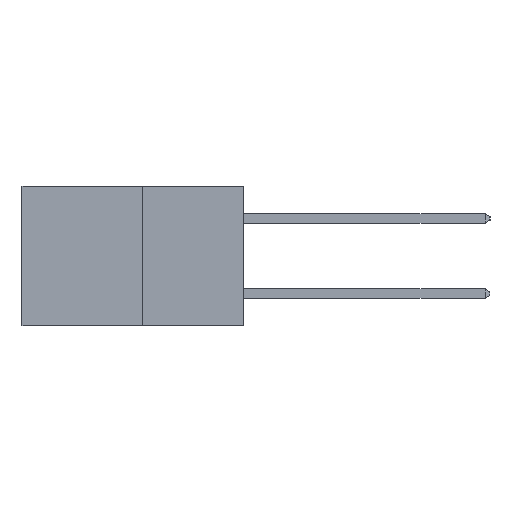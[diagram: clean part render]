
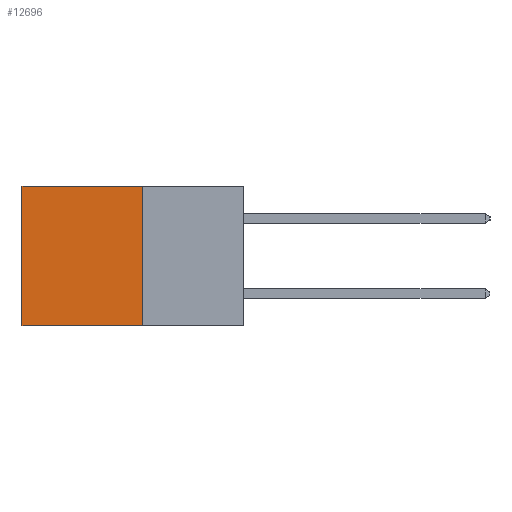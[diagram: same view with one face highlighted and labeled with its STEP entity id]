
A CAD part, left-side view. The second image highlights one B-rep face of the part: STEP entity #12696.
In plain terms, the highlighted planar face has unit normal (-1, 0, 0).
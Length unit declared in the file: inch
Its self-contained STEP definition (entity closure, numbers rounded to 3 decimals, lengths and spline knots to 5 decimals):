
#537 = CARTESIAN_POINT ( 'NONE',  ( 0.277, 0.27, 0. ) ) ;
#1499 = CARTESIAN_POINT ( 'NONE',  ( 0.277, 0.27, -0.37 ) ) ;
#1795 = VERTEX_POINT ( 'NONE', #537 ) ;
#4181 = VECTOR ( 'NONE', #15242, 39.37008 ) ;
#4326 = VECTOR ( 'NONE', #18595, 39.37008 ) ;
#5209 = PLANE ( 'NONE',  #26498 ) ;
#7525 = DIRECTION ( 'NONE',  ( 1., 0., 0. ) ) ;
#9080 = ORIENTED_EDGE ( 'NONE', *, *, #10311, .F. ) ;
#10311 = EDGE_CURVE ( 'NONE', #29391, #19049, #10317, .T. ) ;
#10317 = LINE ( 'NONE', #1499, #4181 ) ;
#11465 = LINE ( 'NONE', #11926, #23617 ) ;
#11926 = CARTESIAN_POINT ( 'NONE',  ( 0.277, 0.59, -0.37 ) ) ;
#12463 = VERTEX_POINT ( 'NONE', #22441 ) ;
#12664 = CARTESIAN_POINT ( 'NONE',  ( 0.277, 0.27, -0.37 ) ) ;
#12682 = CARTESIAN_POINT ( 'NONE',  ( 0.277, 0.59, -0.37 ) ) ;
#12696 = ADVANCED_FACE ( 'NONE', ( #24678 ), #5209, .F. ) ;
#14214 = DIRECTION ( 'NONE',  ( 0., 0., -1. ) ) ;
#14782 = ORIENTED_EDGE ( 'NONE', *, *, #18132, .T. ) ;
#15242 = DIRECTION ( 'NONE',  ( 0., 1., 0. ) ) ;
#16271 = CARTESIAN_POINT ( 'NONE',  ( 0.277, 0.27, 0. ) ) ;
#16441 = EDGE_CURVE ( 'NONE', #1795, #29391, #26967, .T. ) ;
#17982 = LINE ( 'NONE', #16271, #4326 ) ;
#18132 = EDGE_CURVE ( 'NONE', #12463, #19049, #11465, .T. ) ;
#18595 = DIRECTION ( 'NONE',  ( 0., 1., 0. ) ) ;
#19049 = VERTEX_POINT ( 'NONE', #12682 ) ;
#19786 = CARTESIAN_POINT ( 'NONE',  ( 0.277, 0.27, -0.37 ) ) ;
#21252 = CARTESIAN_POINT ( 'NONE',  ( 0.277, 0.27, -0.37 ) ) ;
#22441 = CARTESIAN_POINT ( 'NONE',  ( 0.277, 0.59, 0. ) ) ;
#23516 = DIRECTION ( 'NONE',  ( 0., 0., -1. ) ) ;
#23617 = VECTOR ( 'NONE', #14214, 39.37008 ) ;
#24276 = EDGE_CURVE ( 'NONE', #1795, #12463, #17982, .T. ) ;
#24374 = EDGE_LOOP ( 'NONE', ( #14782, #9080, #24516, #26384 ) ) ;
#24516 = ORIENTED_EDGE ( 'NONE', *, *, #16441, .F. ) ;
#24678 = FACE_OUTER_BOUND ( 'NONE', #24374, .T. ) ;
#25520 = VECTOR ( 'NONE', #26350, 39.37008 ) ;
#26350 = DIRECTION ( 'NONE',  ( 0., 0., -1. ) ) ;
#26384 = ORIENTED_EDGE ( 'NONE', *, *, #24276, .T. ) ;
#26498 = AXIS2_PLACEMENT_3D ( 'NONE', #21252, #7525, #23516 ) ;
#26967 = LINE ( 'NONE', #12664, #25520 ) ;
#29391 = VERTEX_POINT ( 'NONE', #19786 ) ;
